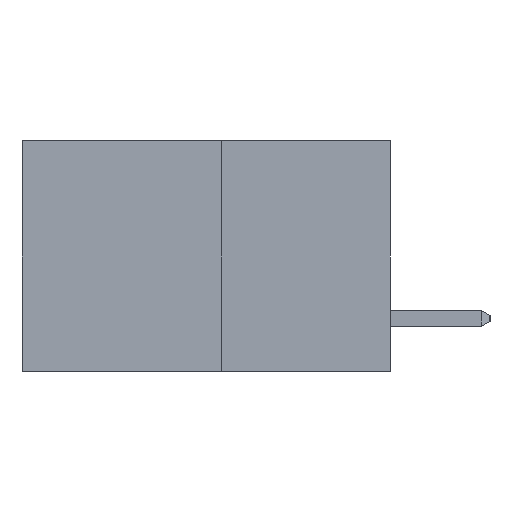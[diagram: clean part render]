
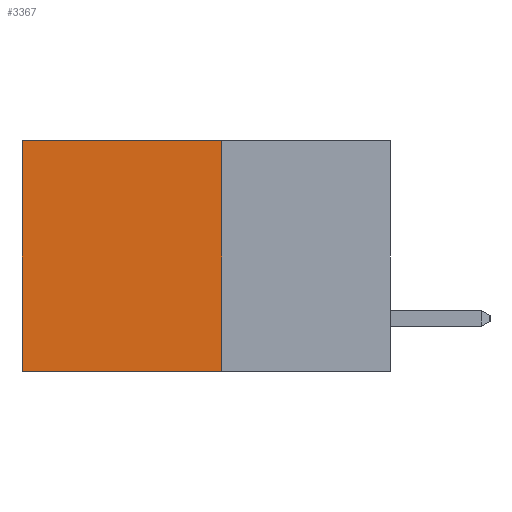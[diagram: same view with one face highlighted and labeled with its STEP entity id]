
A CAD part, left-side view. The second image highlights one B-rep face of the part: STEP entity #3367.
In plain terms, the highlighted planar face has unit normal (-1, 0, 0).
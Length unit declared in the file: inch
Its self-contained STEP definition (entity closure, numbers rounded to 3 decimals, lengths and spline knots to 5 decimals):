
#156 = DIRECTION ( 'NONE',  ( 0., 0., -1. ) ) ;
#187 = DIRECTION ( 'NONE',  ( 1., 0., 0. ) ) ;
#1166 = LINE ( 'NONE', #22551, #6685 ) ;
#1882 = VERTEX_POINT ( 'NONE', #11974 ) ;
#2305 = CARTESIAN_POINT ( 'NONE',  ( 0.277, 0.59, -0.37 ) ) ;
#3367 = ADVANCED_FACE ( 'NONE', ( #14994 ), #4688, .F. ) ;
#3742 = VECTOR ( 'NONE', #11238, 39.37008 ) ;
#3860 = CARTESIAN_POINT ( 'NONE',  ( 0.277, 0.27, 0. ) ) ;
#4688 = PLANE ( 'NONE',  #5002 ) ;
#4856 = EDGE_CURVE ( 'NONE', #21111, #1882, #9537, .T. ) ;
#5002 = AXIS2_PLACEMENT_3D ( 'NONE', #26400, #187, #156 ) ;
#6685 = VECTOR ( 'NONE', #11014, 39.37008 ) ;
#9363 = DIRECTION ( 'NONE',  ( 0., 0., -1. ) ) ;
#9537 = LINE ( 'NONE', #20281, #21853 ) ;
#9995 = LINE ( 'NONE', #22770, #3742 ) ;
#10611 = LINE ( 'NONE', #20894, #16750 ) ;
#10996 = ORIENTED_EDGE ( 'NONE', *, *, #4856, .T. ) ;
#11014 = DIRECTION ( 'NONE',  ( 0., 1., 0. ) ) ;
#11238 = DIRECTION ( 'NONE',  ( 0., 0., -1. ) ) ;
#11974 = CARTESIAN_POINT ( 'NONE',  ( 0.277, 0.59, 0. ) ) ;
#11988 = VERTEX_POINT ( 'NONE', #22406 ) ;
#13461 = EDGE_CURVE ( 'NONE', #1882, #17867, #10611, .T. ) ;
#14994 = FACE_OUTER_BOUND ( 'NONE', #24323, .T. ) ;
#16006 = ORIENTED_EDGE ( 'NONE', *, *, #26651, .F. ) ;
#16750 = VECTOR ( 'NONE', #9363, 39.37008 ) ;
#17710 = EDGE_CURVE ( 'NONE', #21111, #11988, #9995, .T. ) ;
#17867 = VERTEX_POINT ( 'NONE', #2305 ) ;
#18050 = ORIENTED_EDGE ( 'NONE', *, *, #13461, .T. ) ;
#20081 = DIRECTION ( 'NONE',  ( 0., 1., 0. ) ) ;
#20281 = CARTESIAN_POINT ( 'NONE',  ( 0.277, 0.27, 0. ) ) ;
#20894 = CARTESIAN_POINT ( 'NONE',  ( 0.277, 0.59, -0.37 ) ) ;
#21111 = VERTEX_POINT ( 'NONE', #3860 ) ;
#21853 = VECTOR ( 'NONE', #20081, 39.37008 ) ;
#22406 = CARTESIAN_POINT ( 'NONE',  ( 0.277, 0.27, -0.37 ) ) ;
#22551 = CARTESIAN_POINT ( 'NONE',  ( 0.277, 0.27, -0.37 ) ) ;
#22770 = CARTESIAN_POINT ( 'NONE',  ( 0.277, 0.27, -0.37 ) ) ;
#23266 = ORIENTED_EDGE ( 'NONE', *, *, #17710, .F. ) ;
#24323 = EDGE_LOOP ( 'NONE', ( #18050, #16006, #23266, #10996 ) ) ;
#26400 = CARTESIAN_POINT ( 'NONE',  ( 0.277, 0.27, -0.37 ) ) ;
#26651 = EDGE_CURVE ( 'NONE', #11988, #17867, #1166, .T. ) ;
